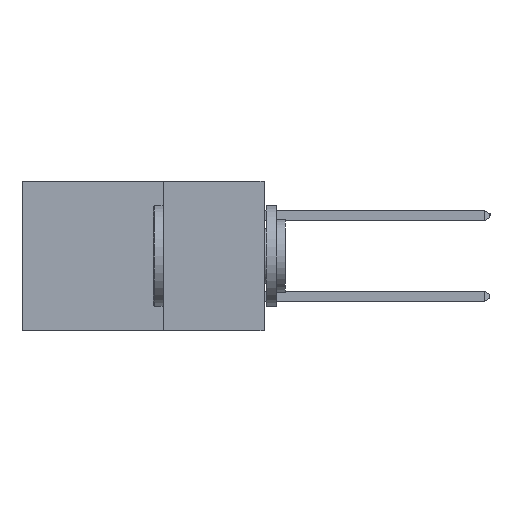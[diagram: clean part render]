
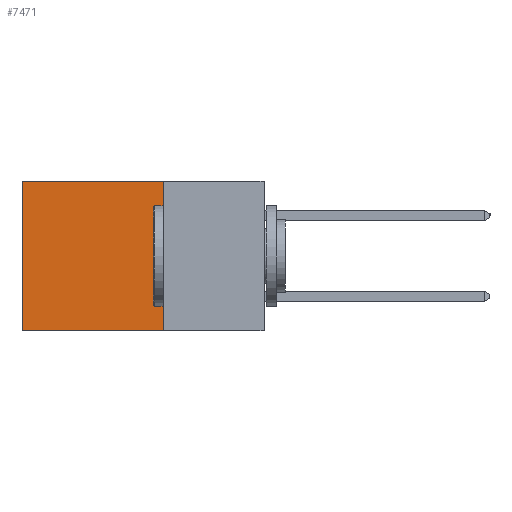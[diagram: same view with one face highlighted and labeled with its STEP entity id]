
A CAD part, left-side view. The second image highlights one B-rep face of the part: STEP entity #7471.
In plain terms, the highlighted planar face has unit normal (-1, 0, 0).
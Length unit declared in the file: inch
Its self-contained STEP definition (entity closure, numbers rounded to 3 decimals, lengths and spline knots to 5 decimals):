
#254 = VECTOR ( 'NONE', #10887, 39.37008 ) ;
#1142 = CARTESIAN_POINT ( 'NONE',  ( 0.2615, 0.6, -0.37 ) ) ;
#1376 = EDGE_CURVE ( 'NONE', #11144, #11284, #7802, .T. ) ;
#1424 = CARTESIAN_POINT ( 'NONE',  ( 0.2615, 0.25, 0. ) ) ;
#2161 = DIRECTION ( 'NONE',  ( 0., 0., -1. ) ) ;
#2174 = LINE ( 'NONE', #8507, #8327 ) ;
#2383 = EDGE_CURVE ( 'NONE', #11284, #12503, #12825, .T. ) ;
#2395 = DIRECTION ( 'NONE',  ( 1., 0., 0. ) ) ;
#3342 = DIRECTION ( 'NONE',  ( 0., 1., 0. ) ) ;
#3574 = PLANE ( 'NONE',  #9270 ) ;
#4630 = DIRECTION ( 'NONE',  ( 0., 0., -1. ) ) ;
#4896 = CARTESIAN_POINT ( 'NONE',  ( 0.2615, 0.25, -0.37 ) ) ;
#5136 = ORIENTED_EDGE ( 'NONE', *, *, #6010, .T. ) ;
#5548 = ORIENTED_EDGE ( 'NONE', *, *, #1376, .F. ) ;
#5854 = VECTOR ( 'NONE', #11771, 39.37008 ) ;
#6010 = EDGE_CURVE ( 'NONE', #11144, #10487, #2174, .T. ) ;
#6391 = ORIENTED_EDGE ( 'NONE', *, *, #8248, .T. ) ;
#6596 = LINE ( 'NONE', #7497, #254 ) ;
#6885 = CARTESIAN_POINT ( 'NONE',  ( 0.2615, 0.6, 0. ) ) ;
#7116 = ORIENTED_EDGE ( 'NONE', *, *, #2383, .F. ) ;
#7471 = ADVANCED_FACE ( 'NONE', ( #9873 ), #3574, .F. ) ;
#7497 = CARTESIAN_POINT ( 'NONE',  ( 0.2615, 0.6, -0.37 ) ) ;
#7530 = EDGE_LOOP ( 'NONE', ( #6391, #7116, #5548, #5136 ) ) ;
#7802 = LINE ( 'NONE', #11944, #8733 ) ;
#8248 = EDGE_CURVE ( 'NONE', #10487, #12503, #6596, .T. ) ;
#8327 = VECTOR ( 'NONE', #3342, 39.37008 ) ;
#8507 = CARTESIAN_POINT ( 'NONE',  ( 0.2615, 0.25, 0. ) ) ;
#8733 = VECTOR ( 'NONE', #2161, 39.37008 ) ;
#9270 = AXIS2_PLACEMENT_3D ( 'NONE', #12045, #2395, #4630 ) ;
#9873 = FACE_OUTER_BOUND ( 'NONE', #7530, .T. ) ;
#10487 = VERTEX_POINT ( 'NONE', #6885 ) ;
#10660 = CARTESIAN_POINT ( 'NONE',  ( 0.2615, 0.25, -0.37 ) ) ;
#10887 = DIRECTION ( 'NONE',  ( 0., 0., -1. ) ) ;
#11144 = VERTEX_POINT ( 'NONE', #1424 ) ;
#11284 = VERTEX_POINT ( 'NONE', #4896 ) ;
#11771 = DIRECTION ( 'NONE',  ( 0., 1., 0. ) ) ;
#11944 = CARTESIAN_POINT ( 'NONE',  ( 0.2615, 0.25, -0.37 ) ) ;
#12045 = CARTESIAN_POINT ( 'NONE',  ( 0.2615, 0.25, -0.37 ) ) ;
#12503 = VERTEX_POINT ( 'NONE', #1142 ) ;
#12825 = LINE ( 'NONE', #10660, #5854 ) ;
